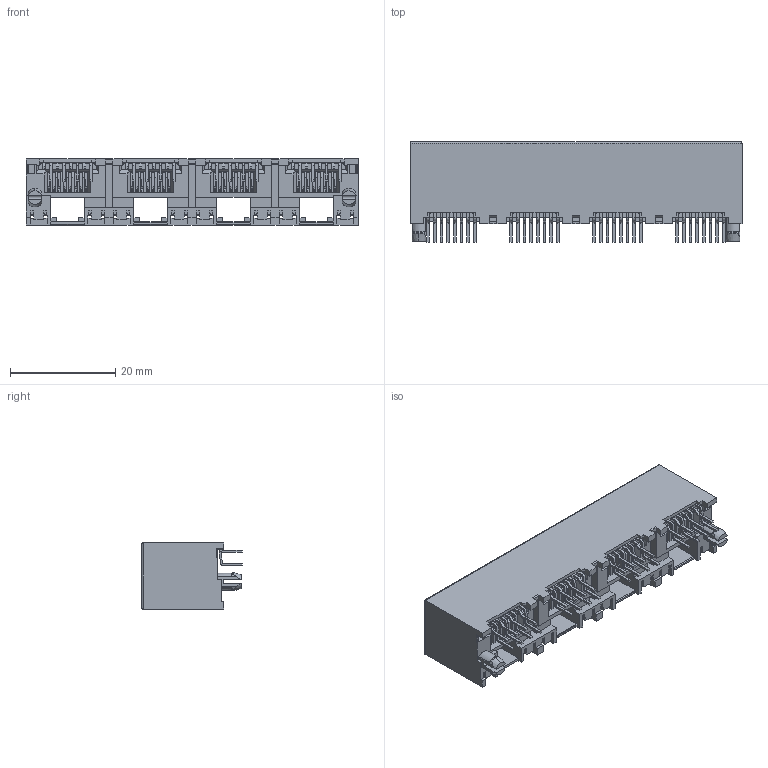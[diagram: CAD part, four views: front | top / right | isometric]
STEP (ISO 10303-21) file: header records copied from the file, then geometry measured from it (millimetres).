
FILE_DESCRIPTION (( 'STEP AP203' ), '1' );
FILE_NAME ('J2W048821N00031.STEP', '2020-10-05T19:54:16', ( '' ), ( '' ), 'SwSTEP 2.0', 'SolidWorks 2020', '' );
FILE_SCHEMA (( 'CONFIG_CONTROL_DESIGN' ));
Length unit declared in the file: millimetre
Products named in the file (6): 2W Contacts; 2W LED RH_0-Blank; J2W048821N00031; 2W Contact Lock; 2W LED LH_0-Blank; 2W Insulator
Assembly tree (9 placements, depth 2):
  2W LED RH_0-Blank
  J2W048821N00031
    2W Insulator
    2W Contacts  x4
    2W Contact Lock  x4
  2W LED LH_0-Blank
Bounding box: 63 x 19.09 x 12.55 mm (x, y, z)
Volume: 5089.9 mm3; surface area: 12247 mm2
Topology: 37 solids, 37 shells, 2879 faces, 8494 edges, 5561 vertices
Faces by surface type: plane 2416, cylinder 405, bspline 47, cone 11
Entity records: 68096 total; most frequent: CARTESIAN_POINT 23536, ORIENTED_EDGE 11114, DIRECTION 6188, EDGE_CURVE 5557, VERTEX_POINT 3623, B_SPLINE_CURVE_WITH_KNOTS 3150, VECTOR 2242, LINE 2242
